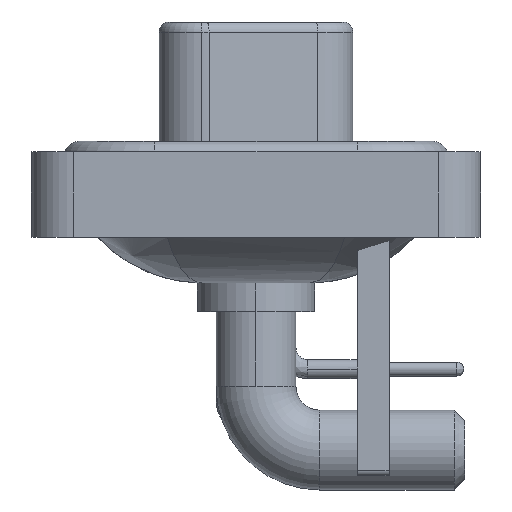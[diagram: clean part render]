
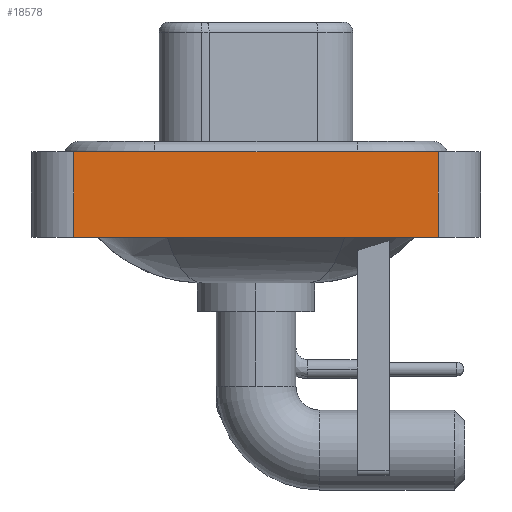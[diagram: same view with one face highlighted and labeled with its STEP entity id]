
A CAD part, left-side view. The second image highlights one B-rep face of the part: STEP entity #18578.
In plain terms, the highlighted planar face has unit normal (-1, 0, 0).
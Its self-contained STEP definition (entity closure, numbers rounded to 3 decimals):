
#1316 = VERTEX_POINT ( 'NONE', #18585 ) ;
#1693 = LINE ( 'NONE', #7847, #10628 ) ;
#2848 = EDGE_LOOP ( 'NONE', ( #20873, #19653, #13168, #23042 ) ) ;
#3108 = LINE ( 'NONE', #10905, #7342 ) ;
#3304 = AXIS2_PLACEMENT_3D ( 'NONE', #17564, #13849, #16026 ) ;
#4241 = EDGE_CURVE ( 'NONE', #1316, #24396, #1693, .T. ) ;
#5574 = CARTESIAN_POINT ( 'NONE',  ( -7.3, -8.55, -3.6 ) ) ;
#6736 = CARTESIAN_POINT ( 'NONE',  ( -7.3, -8.55, 0.4 ) ) ;
#7342 = VECTOR ( 'NONE', #18708, 1000. ) ;
#7700 = DIRECTION ( 'NONE',  ( 0., -1., 0. ) ) ;
#7847 = CARTESIAN_POINT ( 'NONE',  ( -7.3, -8.55, 0.4 ) ) ;
#8745 = LINE ( 'NONE', #14599, #10862 ) ;
#9129 = EDGE_CURVE ( 'NONE', #15795, #23356, #12997, .T. ) ;
#9777 = PLANE ( 'NONE',  #3304 ) ;
#10565 = VECTOR ( 'NONE', #11226, 1000. ) ;
#10628 = VECTOR ( 'NONE', #7700, 1000. ) ;
#10862 = VECTOR ( 'NONE', #22420, 1000. ) ;
#10905 = CARTESIAN_POINT ( 'NONE',  ( -7.3, 8.55, -3.6 ) ) ;
#11226 = DIRECTION ( 'NONE',  ( 0., -1., 0. ) ) ;
#12544 = EDGE_CURVE ( 'NONE', #15795, #1316, #3108, .T. ) ;
#12997 = LINE ( 'NONE', #5574, #10565 ) ;
#13168 = ORIENTED_EDGE ( 'NONE', *, *, #12544, .F. ) ;
#13849 = DIRECTION ( 'NONE',  ( -1., 0., 0. ) ) ;
#14216 = CARTESIAN_POINT ( 'NONE',  ( -7.3, 8.55, -3.6 ) ) ;
#14599 = CARTESIAN_POINT ( 'NONE',  ( -7.3, -8.55, -3.6 ) ) ;
#15795 = VERTEX_POINT ( 'NONE', #14216 ) ;
#16026 = DIRECTION ( 'NONE',  ( 0., 0., 1. ) ) ;
#17564 = CARTESIAN_POINT ( 'NONE',  ( -7.3, -8.55, -3.6 ) ) ;
#17946 = FACE_OUTER_BOUND ( 'NONE', #2848, .T. ) ;
#18578 = ADVANCED_FACE ( 'NONE', ( #17946 ), #9777, .T. ) ;
#18585 = CARTESIAN_POINT ( 'NONE',  ( -7.3, 8.55, 0.4 ) ) ;
#18708 = DIRECTION ( 'NONE',  ( 0., 0., 1. ) ) ;
#19653 = ORIENTED_EDGE ( 'NONE', *, *, #4241, .F. ) ;
#20873 = ORIENTED_EDGE ( 'NONE', *, *, #22252, .T. ) ;
#22252 = EDGE_CURVE ( 'NONE', #23356, #24396, #8745, .T. ) ;
#22420 = DIRECTION ( 'NONE',  ( 0., 0., 1. ) ) ;
#23042 = ORIENTED_EDGE ( 'NONE', *, *, #9129, .T. ) ;
#23356 = VERTEX_POINT ( 'NONE', #25150 ) ;
#24396 = VERTEX_POINT ( 'NONE', #6736 ) ;
#25150 = CARTESIAN_POINT ( 'NONE',  ( -7.3, -8.55, -3.6 ) ) ;
